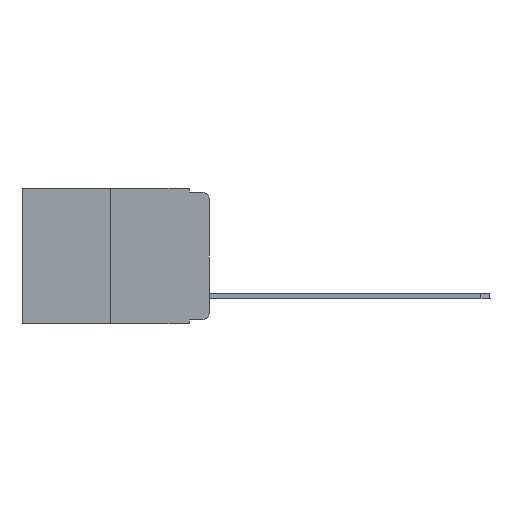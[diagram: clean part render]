
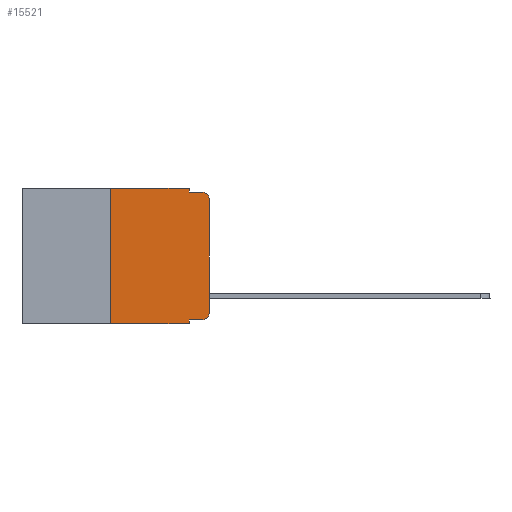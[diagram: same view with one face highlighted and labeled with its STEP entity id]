
A CAD part, left-side view. The second image highlights one B-rep face of the part: STEP entity #15521.
In plain terms, the highlighted planar face has unit normal (-1, 0, 0).
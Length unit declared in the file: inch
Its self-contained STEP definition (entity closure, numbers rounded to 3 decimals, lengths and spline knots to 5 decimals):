
#173 = PLANE ( 'NONE',  #13304 ) ;
#1865 = CARTESIAN_POINT ( 'NONE',  ( 0., 0.051, -0.01 ) ) ;
#1935 = CARTESIAN_POINT ( 'NONE',  ( 0., 0.051, 0. ) ) ;
#2113 = ORIENTED_EDGE ( 'NONE', *, *, #18599, .F. ) ;
#2696 = VERTEX_POINT ( 'NONE', #11402 ) ;
#2872 = EDGE_CURVE ( 'NONE', #23469, #17880, #10905, .T. ) ;
#3186 = CIRCLE ( 'NONE', #6321, 0.02 ) ;
#3479 = EDGE_CURVE ( 'NONE', #3994, #2696, #21914, .T. ) ;
#3853 = VERTEX_POINT ( 'NONE', #16116 ) ;
#3994 = VERTEX_POINT ( 'NONE', #1865 ) ;
#4496 = ORIENTED_EDGE ( 'NONE', *, *, #6554, .T. ) ;
#4508 = ORIENTED_EDGE ( 'NONE', *, *, #9936, .F. ) ;
#4719 = DIRECTION ( 'NONE',  ( 0., 0., -1. ) ) ;
#5621 = CARTESIAN_POINT ( 'NONE',  ( 0., 0.051, -0.333 ) ) ;
#6051 = DIRECTION ( 'NONE',  ( 0., 0., -1. ) ) ;
#6207 = LINE ( 'NONE', #5621, #12884 ) ;
#6267 = EDGE_LOOP ( 'NONE', ( #9568, #6537, #22095, #17304, #19628, #2113, #17822, #4508, #4496, #22217 ) ) ;
#6321 = AXIS2_PLACEMENT_3D ( 'NONE', #15867, #6545, #19573 ) ;
#6537 = ORIENTED_EDGE ( 'NONE', *, *, #14782, .T. ) ;
#6545 = DIRECTION ( 'NONE',  ( -1., 0., 0. ) ) ;
#6554 = EDGE_CURVE ( 'NONE', #3853, #8919, #6207, .T. ) ;
#7192 = DIRECTION ( 'NONE',  ( 0., -1., 0. ) ) ;
#7514 = DIRECTION ( 'NONE',  ( 0., 0., -1. ) ) ;
#8043 = CARTESIAN_POINT ( 'NONE',  ( 0., 0.25, 0. ) ) ;
#8194 = VECTOR ( 'NONE', #23741, 39.37008 ) ;
#8919 = VERTEX_POINT ( 'NONE', #12774 ) ;
#8935 = CARTESIAN_POINT ( 'NONE',  ( 0., 0.051, -0.01 ) ) ;
#9549 = EDGE_CURVE ( 'NONE', #8919, #16825, #18588, .T. ) ;
#9568 = ORIENTED_EDGE ( 'NONE', *, *, #15116, .T. ) ;
#9936 = EDGE_CURVE ( 'NONE', #3853, #17880, #22684, .T. ) ;
#10188 = DIRECTION ( 'NONE',  ( 0., -1., 0. ) ) ;
#10905 = LINE ( 'NONE', #17333, #22867 ) ;
#11402 = CARTESIAN_POINT ( 'NONE',  ( 0., 0.02, -0.01 ) ) ;
#11869 = LINE ( 'NONE', #16995, #23585 ) ;
#12464 = CARTESIAN_POINT ( 'NONE',  ( 0., 0.25, -0.343 ) ) ;
#12774 = CARTESIAN_POINT ( 'NONE',  ( 0., 0.02, -0.333 ) ) ;
#12884 = VECTOR ( 'NONE', #14692, 39.37008 ) ;
#12886 = CARTESIAN_POINT ( 'NONE',  ( 0., 0.25, 0. ) ) ;
#13195 = VERTEX_POINT ( 'NONE', #16282 ) ;
#13304 = AXIS2_PLACEMENT_3D ( 'NONE', #20918, #20847, #19222 ) ;
#13435 = FACE_OUTER_BOUND ( 'NONE', #6267, .T. ) ;
#13899 = CARTESIAN_POINT ( 'NONE',  ( 0., 0., -0.313 ) ) ;
#13901 = VERTEX_POINT ( 'NONE', #16421 ) ;
#13948 = CARTESIAN_POINT ( 'NONE',  ( 0., 0.051, 0. ) ) ;
#14692 = DIRECTION ( 'NONE',  ( 0., -1., 0. ) ) ;
#14782 = EDGE_CURVE ( 'NONE', #13901, #2696, #3186, .T. ) ;
#14842 = LINE ( 'NONE', #13948, #15138 ) ;
#14861 = LINE ( 'NONE', #8043, #20736 ) ;
#15116 = EDGE_CURVE ( 'NONE', #16825, #13901, #11869, .T. ) ;
#15138 = VECTOR ( 'NONE', #4719, 39.37008 ) ;
#15521 = ADVANCED_FACE ( 'NONE', ( #13435 ), #173, .F. ) ;
#15867 = CARTESIAN_POINT ( 'NONE',  ( 0., 0.02, -0.03 ) ) ;
#15929 = VECTOR ( 'NONE', #7514, 39.37008 ) ;
#16116 = CARTESIAN_POINT ( 'NONE',  ( 0., 0.051, -0.333 ) ) ;
#16282 = CARTESIAN_POINT ( 'NONE',  ( 0., 0.051, 0. ) ) ;
#16421 = CARTESIAN_POINT ( 'NONE',  ( 0., 0., -0.03 ) ) ;
#16825 = VERTEX_POINT ( 'NONE', #13899 ) ;
#16995 = CARTESIAN_POINT ( 'NONE',  ( 0., 0., 0. ) ) ;
#17147 = VERTEX_POINT ( 'NONE', #12886 ) ;
#17304 = ORIENTED_EDGE ( 'NONE', *, *, #18944, .F. ) ;
#17333 = CARTESIAN_POINT ( 'NONE',  ( 0., 0.473, -0.343 ) ) ;
#17437 = VECTOR ( 'NONE', #7192, 39.37008 ) ;
#17822 = ORIENTED_EDGE ( 'NONE', *, *, #2872, .T. ) ;
#17880 = VERTEX_POINT ( 'NONE', #19291 ) ;
#18588 = CIRCLE ( 'NONE', #18886, 0.02 ) ;
#18599 = EDGE_CURVE ( 'NONE', #23469, #17147, #14861, .T. ) ;
#18886 = AXIS2_PLACEMENT_3D ( 'NONE', #20884, #20964, #6051 ) ;
#18944 = EDGE_CURVE ( 'NONE', #13195, #3994, #14842, .T. ) ;
#19222 = DIRECTION ( 'NONE',  ( 0., 0., -1. ) ) ;
#19291 = CARTESIAN_POINT ( 'NONE',  ( 0., 0.051, -0.343 ) ) ;
#19573 = DIRECTION ( 'NONE',  ( 0., 0., -1. ) ) ;
#19628 = ORIENTED_EDGE ( 'NONE', *, *, #19801, .F. ) ;
#19801 = EDGE_CURVE ( 'NONE', #17147, #13195, #21262, .T. ) ;
#20233 = CARTESIAN_POINT ( 'NONE',  ( 0., 0.473, 0. ) ) ;
#20736 = VECTOR ( 'NONE', #21076, 39.37008 ) ;
#20847 = DIRECTION ( 'NONE',  ( 1., 0., 0. ) ) ;
#20884 = CARTESIAN_POINT ( 'NONE',  ( 0., 0.02, -0.313 ) ) ;
#20918 = CARTESIAN_POINT ( 'NONE',  ( 0., 0.473, 0. ) ) ;
#20964 = DIRECTION ( 'NONE',  ( -1., 0., 0. ) ) ;
#21076 = DIRECTION ( 'NONE',  ( 0., 0., 1. ) ) ;
#21262 = LINE ( 'NONE', #20233, #17437 ) ;
#21914 = LINE ( 'NONE', #8935, #8194 ) ;
#22095 = ORIENTED_EDGE ( 'NONE', *, *, #3479, .F. ) ;
#22217 = ORIENTED_EDGE ( 'NONE', *, *, #9549, .T. ) ;
#22684 = LINE ( 'NONE', #1935, #15929 ) ;
#22740 = DIRECTION ( 'NONE',  ( 0., 0., 1. ) ) ;
#22867 = VECTOR ( 'NONE', #10188, 39.37008 ) ;
#23469 = VERTEX_POINT ( 'NONE', #12464 ) ;
#23585 = VECTOR ( 'NONE', #22740, 39.37008 ) ;
#23741 = DIRECTION ( 'NONE',  ( 0., -1., 0. ) ) ;
